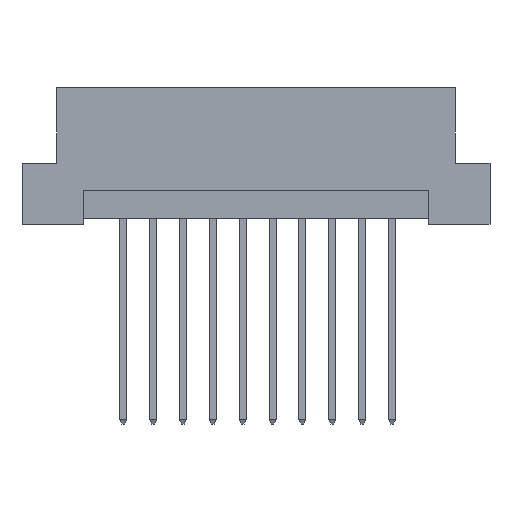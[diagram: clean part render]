
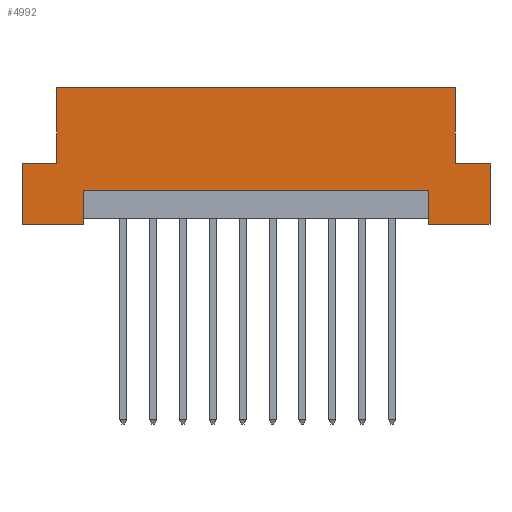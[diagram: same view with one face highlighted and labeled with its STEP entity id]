
A CAD part, front view. The second image highlights one B-rep face of the part: STEP entity #4992.
In plain terms, the highlighted planar face has unit normal (0, -1, 0).
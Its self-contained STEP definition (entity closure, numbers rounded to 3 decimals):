
#17 = CARTESIAN_POINT ( 'NONE',  ( 19.9, 0., 0. ) ) ;
#91 = VERTEX_POINT ( 'NONE', #4650 ) ;
#235 = LINE ( 'NONE', #3158, #1715 ) ;
#241 = DIRECTION ( 'NONE',  ( 1., 0., 0. ) ) ;
#316 = CARTESIAN_POINT ( 'NONE',  ( -19.9, 0., 5.2 ) ) ;
#319 = EDGE_CURVE ( 'NONE', #2650, #773, #4975, .T. ) ;
#334 = LINE ( 'NONE', #4821, #729 ) ;
#435 = CARTESIAN_POINT ( 'NONE',  ( -19.9, 0., 0. ) ) ;
#554 = ORIENTED_EDGE ( 'NONE', *, *, #6506, .F. ) ;
#695 = VERTEX_POINT ( 'NONE', #3231 ) ;
#697 = CARTESIAN_POINT ( 'NONE',  ( -14.69, 0., 2.9 ) ) ;
#729 = VECTOR ( 'NONE', #4296, 1000. ) ;
#773 = VERTEX_POINT ( 'NONE', #1631 ) ;
#939 = LINE ( 'NONE', #316, #5216 ) ;
#944 = ORIENTED_EDGE ( 'NONE', *, *, #319, .T. ) ;
#977 = CARTESIAN_POINT ( 'NONE',  ( -19.9, 0., 5.2 ) ) ;
#1030 = CARTESIAN_POINT ( 'NONE',  ( -19.9, 0., 0. ) ) ;
#1254 = VECTOR ( 'NONE', #6741, 1000. ) ;
#1414 = ORIENTED_EDGE ( 'NONE', *, *, #6087, .F. ) ;
#1454 = VECTOR ( 'NONE', #2747, 1000. ) ;
#1631 = CARTESIAN_POINT ( 'NONE',  ( 14.69, 0., 0. ) ) ;
#1678 = LINE ( 'NONE', #4527, #6088 ) ;
#1715 = VECTOR ( 'NONE', #5420, 1000. ) ;
#1818 = EDGE_LOOP ( 'NONE', ( #7159, #944, #6379, #1414, #554, #5909, #6884, #3088, #6649, #3966, #5155, #7283 ) ) ;
#1905 = LINE ( 'NONE', #3720, #4445 ) ;
#2114 = DIRECTION ( 'NONE',  ( -1., 0., 0. ) ) ;
#2280 = VECTOR ( 'NONE', #4648, 1000. ) ;
#2305 = EDGE_CURVE ( 'NONE', #3003, #2765, #2672, .T. ) ;
#2557 = VECTOR ( 'NONE', #6793, 1000. ) ;
#2650 = VERTEX_POINT ( 'NONE', #6018 ) ;
#2672 = LINE ( 'NONE', #5522, #6944 ) ;
#2747 = DIRECTION ( 'NONE',  ( -1., 0., 0. ) ) ;
#2765 = VERTEX_POINT ( 'NONE', #1030 ) ;
#2833 = LINE ( 'NONE', #5094, #6653 ) ;
#3003 = VERTEX_POINT ( 'NONE', #5319 ) ;
#3020 = CARTESIAN_POINT ( 'NONE',  ( 16.94, 0., 11.6 ) ) ;
#3083 = CARTESIAN_POINT ( 'NONE',  ( 19.9, 0., 0. ) ) ;
#3088 = ORIENTED_EDGE ( 'NONE', *, *, #6969, .F. ) ;
#3090 = CARTESIAN_POINT ( 'NONE',  ( -19.9, 0., 11.6 ) ) ;
#3158 = CARTESIAN_POINT ( 'NONE',  ( -16.94, 0., 5.2 ) ) ;
#3231 = CARTESIAN_POINT ( 'NONE',  ( 16.94, 0., 5.2 ) ) ;
#3488 = VERTEX_POINT ( 'NONE', #697 ) ;
#3720 = CARTESIAN_POINT ( 'NONE',  ( -14.69, 0., 0.5 ) ) ;
#3779 = CARTESIAN_POINT ( 'NONE',  ( -16.94, 0., 11.6 ) ) ;
#3917 = LINE ( 'NONE', #17, #5514 ) ;
#3966 = ORIENTED_EDGE ( 'NONE', *, *, #6158, .F. ) ;
#4024 = AXIS2_PLACEMENT_3D ( 'NONE', #3090, #4838, #4763 ) ;
#4126 = EDGE_CURVE ( 'NONE', #2650, #3488, #334, .T. ) ;
#4238 = PLANE ( 'NONE',  #4024 ) ;
#4278 = LINE ( 'NONE', #435, #2557 ) ;
#4296 = DIRECTION ( 'NONE',  ( -1., 0., 0. ) ) ;
#4445 = VECTOR ( 'NONE', #6549, 1000. ) ;
#4512 = VERTEX_POINT ( 'NONE', #3779 ) ;
#4527 = CARTESIAN_POINT ( 'NONE',  ( 19.9, 0., 5.2 ) ) ;
#4648 = DIRECTION ( 'NONE',  ( 1., 0., 0. ) ) ;
#4650 = CARTESIAN_POINT ( 'NONE',  ( 19.9, 0., 5.2 ) ) ;
#4688 = EDGE_CURVE ( 'NONE', #695, #5417, #2833, .T. ) ;
#4763 = DIRECTION ( 'NONE',  ( 0., 0., 1. ) ) ;
#4821 = CARTESIAN_POINT ( 'NONE',  ( 14.69, 0., 2.9 ) ) ;
#4838 = DIRECTION ( 'NONE',  ( 0., 1., 0. ) ) ;
#4870 = CARTESIAN_POINT ( 'NONE',  ( -16.94, 0., 5.2 ) ) ;
#4975 = LINE ( 'NONE', #7140, #1254 ) ;
#4981 = EDGE_CURVE ( 'NONE', #6627, #7028, #939, .T. ) ;
#4992 = ADVANCED_FACE ( 'NONE', ( #6000 ), #4238, .F. ) ;
#5094 = CARTESIAN_POINT ( 'NONE',  ( 16.94, 0., 5.2 ) ) ;
#5155 = ORIENTED_EDGE ( 'NONE', *, *, #2305, .F. ) ;
#5216 = VECTOR ( 'NONE', #241, 1000. ) ;
#5277 = LINE ( 'NONE', #5802, #2280 ) ;
#5319 = CARTESIAN_POINT ( 'NONE',  ( -14.69, 0., 0. ) ) ;
#5417 = VERTEX_POINT ( 'NONE', #3020 ) ;
#5420 = DIRECTION ( 'NONE',  ( 0., 0., 1. ) ) ;
#5514 = VECTOR ( 'NONE', #6155, 1000. ) ;
#5522 = CARTESIAN_POINT ( 'NONE',  ( -19.9, 0., 0. ) ) ;
#5645 = CARTESIAN_POINT ( 'NONE',  ( -19.9, 0., 0. ) ) ;
#5802 = CARTESIAN_POINT ( 'NONE',  ( -19.9, 0., 11.6 ) ) ;
#5909 = ORIENTED_EDGE ( 'NONE', *, *, #4688, .T. ) ;
#6000 = FACE_OUTER_BOUND ( 'NONE', #1818, .T. ) ;
#6018 = CARTESIAN_POINT ( 'NONE',  ( 14.69, 0., 2.9 ) ) ;
#6087 = EDGE_CURVE ( 'NONE', #91, #6961, #3917, .T. ) ;
#6088 = VECTOR ( 'NONE', #6147, 1000. ) ;
#6124 = DIRECTION ( 'NONE',  ( 0., 0., 1. ) ) ;
#6147 = DIRECTION ( 'NONE',  ( 1., 0., 0. ) ) ;
#6155 = DIRECTION ( 'NONE',  ( 0., 0., -1. ) ) ;
#6158 = EDGE_CURVE ( 'NONE', #2765, #6627, #4278, .T. ) ;
#6379 = ORIENTED_EDGE ( 'NONE', *, *, #6492, .F. ) ;
#6492 = EDGE_CURVE ( 'NONE', #6961, #773, #7268, .T. ) ;
#6506 = EDGE_CURVE ( 'NONE', #695, #91, #1678, .T. ) ;
#6549 = DIRECTION ( 'NONE',  ( 0., 0., -1. ) ) ;
#6627 = VERTEX_POINT ( 'NONE', #977 ) ;
#6649 = ORIENTED_EDGE ( 'NONE', *, *, #4981, .F. ) ;
#6653 = VECTOR ( 'NONE', #6124, 1000. ) ;
#6741 = DIRECTION ( 'NONE',  ( 0., 0., -1. ) ) ;
#6781 = EDGE_CURVE ( 'NONE', #4512, #5417, #5277, .T. ) ;
#6793 = DIRECTION ( 'NONE',  ( 0., 0., 1. ) ) ;
#6884 = ORIENTED_EDGE ( 'NONE', *, *, #6781, .F. ) ;
#6944 = VECTOR ( 'NONE', #2114, 1000. ) ;
#6961 = VERTEX_POINT ( 'NONE', #3083 ) ;
#6969 = EDGE_CURVE ( 'NONE', #7028, #4512, #235, .T. ) ;
#7005 = EDGE_CURVE ( 'NONE', #3488, #3003, #1905, .T. ) ;
#7028 = VERTEX_POINT ( 'NONE', #4870 ) ;
#7140 = CARTESIAN_POINT ( 'NONE',  ( 14.69, 0., 0.5 ) ) ;
#7159 = ORIENTED_EDGE ( 'NONE', *, *, #4126, .F. ) ;
#7268 = LINE ( 'NONE', #5645, #1454 ) ;
#7283 = ORIENTED_EDGE ( 'NONE', *, *, #7005, .F. ) ;
